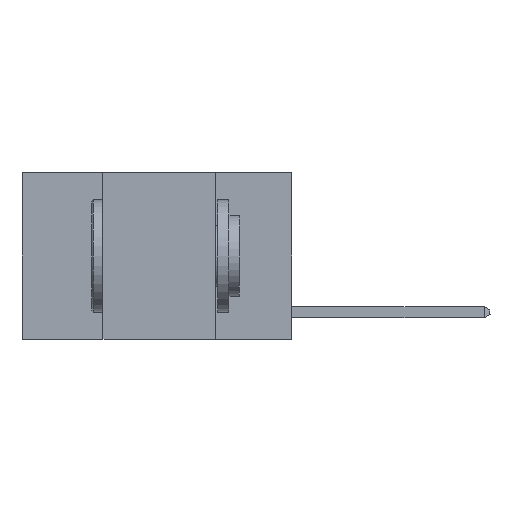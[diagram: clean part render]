
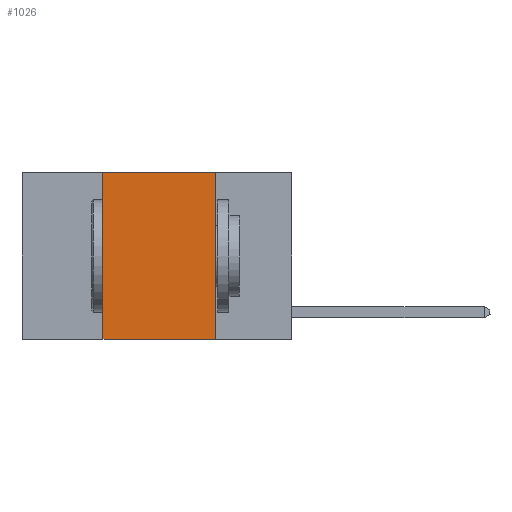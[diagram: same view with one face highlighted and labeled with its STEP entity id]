
A CAD part, left-side view. The second image highlights one B-rep face of the part: STEP entity #1026.
In plain terms, the highlighted planar face has unit normal (-1, 0, 0).
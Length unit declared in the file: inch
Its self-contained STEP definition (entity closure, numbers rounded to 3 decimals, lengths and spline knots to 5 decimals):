
#292 = ORIENTED_EDGE ( 'NONE', *, *, #2136, .T. ) ;
#961 = EDGE_CURVE ( 'NONE', #10608, #13174, #10808, .T. ) ;
#1015 = CARTESIAN_POINT ( 'NONE',  ( 0., 0.6, -0.37 ) ) ;
#1026 = ADVANCED_FACE ( 'NONE', ( #18737 ), #11764, .F. ) ;
#1216 = CARTESIAN_POINT ( 'NONE',  ( 0., 0.42, 0. ) ) ;
#1424 = DIRECTION ( 'NONE',  ( 0., -1., 0. ) ) ;
#1975 = DIRECTION ( 'NONE',  ( 0., 0., -1. ) ) ;
#2136 = EDGE_CURVE ( 'NONE', #15835, #15449, #3211, .T. ) ;
#2950 = DIRECTION ( 'NONE',  ( 0., 0., 1. ) ) ;
#3211 = LINE ( 'NONE', #1015, #7158 ) ;
#3306 = CARTESIAN_POINT ( 'NONE',  ( 0., 0.17, 0. ) ) ;
#4798 = EDGE_LOOP ( 'NONE', ( #16547, #8371, #15951, #292 ) ) ;
#6005 = EDGE_CURVE ( 'NONE', #13174, #15449, #16948, .T. ) ;
#7158 = VECTOR ( 'NONE', #1424, 39.37008 ) ;
#7773 = DIRECTION ( 'NONE',  ( 0., -1., 0. ) ) ;
#7818 = VECTOR ( 'NONE', #13594, 39.37008 ) ;
#8371 = ORIENTED_EDGE ( 'NONE', *, *, #961, .F. ) ;
#8757 = AXIS2_PLACEMENT_3D ( 'NONE', #20185, #18699, #1975 ) ;
#9613 = CARTESIAN_POINT ( 'NONE',  ( 0., 0.17, -0.37 ) ) ;
#10061 = CARTESIAN_POINT ( 'NONE',  ( 0., 0.6, 0. ) ) ;
#10547 = CARTESIAN_POINT ( 'NONE',  ( 0., 0.42, 0. ) ) ;
#10608 = VERTEX_POINT ( 'NONE', #10547 ) ;
#10808 = LINE ( 'NONE', #10061, #19252 ) ;
#11764 = PLANE ( 'NONE',  #8757 ) ;
#12119 = VECTOR ( 'NONE', #2950, 39.37008 ) ;
#13174 = VERTEX_POINT ( 'NONE', #13612 ) ;
#13594 = DIRECTION ( 'NONE',  ( 0., 0., -1. ) ) ;
#13612 = CARTESIAN_POINT ( 'NONE',  ( 0., 0.17, 0. ) ) ;
#15449 = VERTEX_POINT ( 'NONE', #9613 ) ;
#15835 = VERTEX_POINT ( 'NONE', #20678 ) ;
#15951 = ORIENTED_EDGE ( 'NONE', *, *, #18589, .F. ) ;
#16547 = ORIENTED_EDGE ( 'NONE', *, *, #6005, .F. ) ;
#16948 = LINE ( 'NONE', #3306, #7818 ) ;
#18589 = EDGE_CURVE ( 'NONE', #15835, #10608, #21008, .T. ) ;
#18699 = DIRECTION ( 'NONE',  ( 1., 0., 0. ) ) ;
#18737 = FACE_OUTER_BOUND ( 'NONE', #4798, .T. ) ;
#19252 = VECTOR ( 'NONE', #7773, 39.37008 ) ;
#20185 = CARTESIAN_POINT ( 'NONE',  ( 0., 0.6, 0. ) ) ;
#20678 = CARTESIAN_POINT ( 'NONE',  ( 0., 0.42, -0.37 ) ) ;
#21008 = LINE ( 'NONE', #1216, #12119 ) ;
